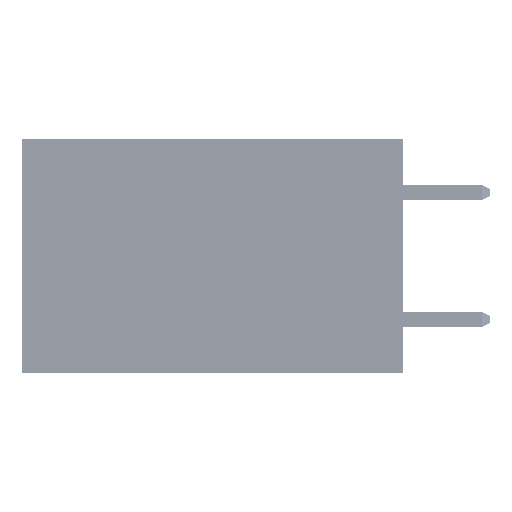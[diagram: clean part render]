
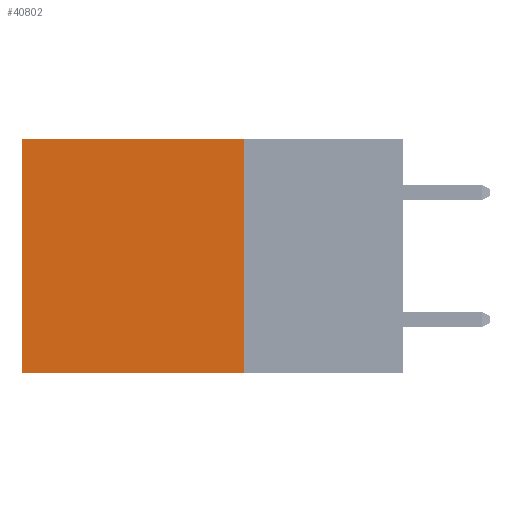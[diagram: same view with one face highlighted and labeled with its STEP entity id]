
A CAD part, left-side view. The second image highlights one B-rep face of the part: STEP entity #40802.
In plain terms, the highlighted planar face has unit normal (-1, 0, 0).
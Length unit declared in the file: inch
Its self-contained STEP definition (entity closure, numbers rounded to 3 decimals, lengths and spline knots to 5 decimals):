
#593 = PLANE ( 'NONE',  #23911 ) ;
#824 = CARTESIAN_POINT ( 'NONE',  ( 0.2875, 0.25, -0.37 ) ) ;
#1184 = CARTESIAN_POINT ( 'NONE',  ( 0.2875, 0.25, 0. ) ) ;
#2745 = VECTOR ( 'NONE', #49900, 39.37008 ) ;
#3650 = VECTOR ( 'NONE', #50524, 39.37008 ) ;
#4732 = CARTESIAN_POINT ( 'NONE',  ( 0.2875, 0.25, 0. ) ) ;
#5688 = EDGE_CURVE ( 'NONE', #16629, #9231, #36704, .T. ) ;
#9231 = VERTEX_POINT ( 'NONE', #13582 ) ;
#9364 = DIRECTION ( 'NONE',  ( 0., 0., -1. ) ) ;
#13213 = VECTOR ( 'NONE', #21218, 39.37008 ) ;
#13582 = CARTESIAN_POINT ( 'NONE',  ( 0.2875, 0.6, -0.37 ) ) ;
#14189 = VECTOR ( 'NONE', #21827, 39.37008 ) ;
#14199 = CARTESIAN_POINT ( 'NONE',  ( 0.2875, 0.25, 0. ) ) ;
#16629 = VERTEX_POINT ( 'NONE', #824 ) ;
#17216 = EDGE_LOOP ( 'NONE', ( #21172, #39030, #38379, #38451 ) ) ;
#20977 = FACE_OUTER_BOUND ( 'NONE', #17216, .T. ) ;
#21172 = ORIENTED_EDGE ( 'NONE', *, *, #30515, .T. ) ;
#21218 = DIRECTION ( 'NONE',  ( 0., 1., 0. ) ) ;
#21827 = DIRECTION ( 'NONE',  ( 0., 1., 0. ) ) ;
#23911 = AXIS2_PLACEMENT_3D ( 'NONE', #4732, #44728, #9364 ) ;
#25893 = LINE ( 'NONE', #41653, #2745 ) ;
#27050 = VERTEX_POINT ( 'NONE', #47501 ) ;
#30515 = EDGE_CURVE ( 'NONE', #27050, #9231, #34504, .T. ) ;
#33076 = CARTESIAN_POINT ( 'NONE',  ( 0.2875, 0.25, -0.37 ) ) ;
#33422 = LINE ( 'NONE', #1184, #14189 ) ;
#34504 = LINE ( 'NONE', #50780, #3650 ) ;
#36704 = LINE ( 'NONE', #33076, #13213 ) ;
#38379 = ORIENTED_EDGE ( 'NONE', *, *, #46831, .F. ) ;
#38451 = ORIENTED_EDGE ( 'NONE', *, *, #43565, .T. ) ;
#39030 = ORIENTED_EDGE ( 'NONE', *, *, #5688, .F. ) ;
#40802 = ADVANCED_FACE ( 'NONE', ( #20977 ), #593, .F. ) ;
#41364 = VERTEX_POINT ( 'NONE', #14199 ) ;
#41653 = CARTESIAN_POINT ( 'NONE',  ( 0.2875, 0.25, 0. ) ) ;
#43565 = EDGE_CURVE ( 'NONE', #41364, #27050, #33422, .T. ) ;
#44728 = DIRECTION ( 'NONE',  ( 1., 0., 0. ) ) ;
#46831 = EDGE_CURVE ( 'NONE', #41364, #16629, #25893, .T. ) ;
#47501 = CARTESIAN_POINT ( 'NONE',  ( 0.2875, 0.6, 0. ) ) ;
#49900 = DIRECTION ( 'NONE',  ( 0., 0., -1. ) ) ;
#50524 = DIRECTION ( 'NONE',  ( 0., 0., -1. ) ) ;
#50780 = CARTESIAN_POINT ( 'NONE',  ( 0.2875, 0.6, 0. ) ) ;
